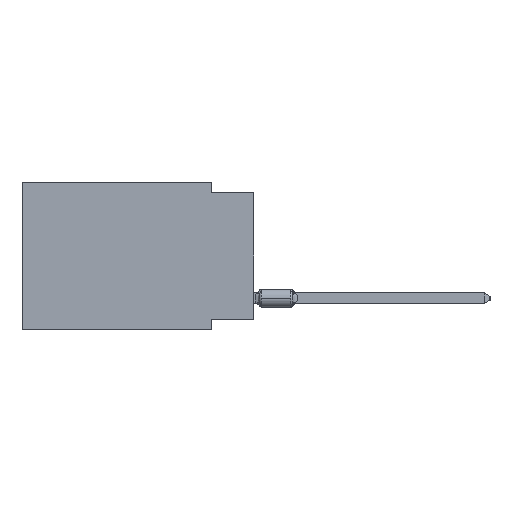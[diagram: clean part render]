
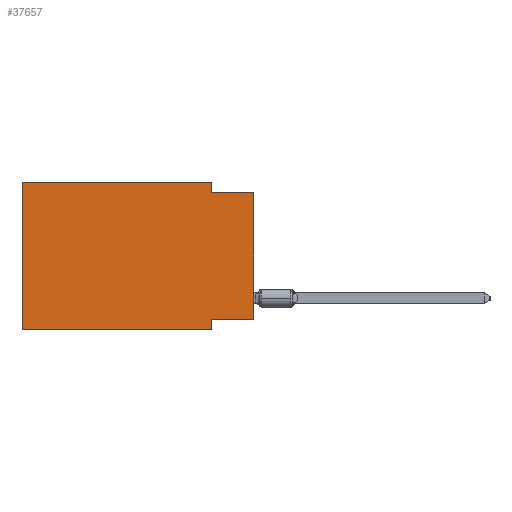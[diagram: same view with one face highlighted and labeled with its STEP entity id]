
A CAD part, left-side view. The second image highlights one B-rep face of the part: STEP entity #37657.
In plain terms, the highlighted planar face has unit normal (-1, 0, 0).
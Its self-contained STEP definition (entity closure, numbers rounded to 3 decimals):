
#458 = EDGE_CURVE ( 'NONE', #14854, #29812, #41753, .T. ) ;
#502 = ORIENTED_EDGE ( 'NONE', *, *, #43534, .T. ) ;
#1243 = CARTESIAN_POINT ( 'NONE',  ( 0., 2.54, -8.255 ) ) ;
#1617 = LINE ( 'NONE', #15520, #10280 ) ;
#2071 = VECTOR ( 'NONE', #35717, 1000. ) ;
#2392 = VERTEX_POINT ( 'NONE', #25426 ) ;
#7444 = VECTOR ( 'NONE', #23663, 1000. ) ;
#8389 = EDGE_CURVE ( 'NONE', #2392, #30727, #14207, .T. ) ;
#8880 = ORIENTED_EDGE ( 'NONE', *, *, #15803, .T. ) ;
#9015 = VECTOR ( 'NONE', #29003, 1000. ) ;
#9169 = VERTEX_POINT ( 'NONE', #44141 ) ;
#9697 = VERTEX_POINT ( 'NONE', #14405 ) ;
#10077 = CARTESIAN_POINT ( 'NONE',  ( 0., 0., -0.635 ) ) ;
#10280 = VECTOR ( 'NONE', #29429, 1000. ) ;
#10517 = CARTESIAN_POINT ( 'NONE',  ( 0., 2.54, -8.89 ) ) ;
#11199 = ORIENTED_EDGE ( 'NONE', *, *, #38342, .F. ) ;
#11310 = DIRECTION ( 'NONE',  ( 1., 0., 0. ) ) ;
#11947 = VERTEX_POINT ( 'NONE', #10077 ) ;
#12140 = DIRECTION ( 'NONE',  ( 0., 0., -1. ) ) ;
#12827 = ORIENTED_EDGE ( 'NONE', *, *, #37064, .F. ) ;
#14122 = VERTEX_POINT ( 'NONE', #43372 ) ;
#14207 = LINE ( 'NONE', #21698, #28660 ) ;
#14405 = CARTESIAN_POINT ( 'NONE',  ( 0., 13.97, -8.89 ) ) ;
#14854 = VERTEX_POINT ( 'NONE', #1243 ) ;
#15520 = CARTESIAN_POINT ( 'NONE',  ( 0., 13.97, 0. ) ) ;
#15803 = EDGE_CURVE ( 'NONE', #9697, #29812, #36028, .T. ) ;
#16454 = LINE ( 'NONE', #16675, #33556 ) ;
#16675 = CARTESIAN_POINT ( 'NONE',  ( 0., 0., -8.255 ) ) ;
#17127 = DIRECTION ( 'NONE',  ( 0., 0., -1. ) ) ;
#18142 = LINE ( 'NONE', #42327, #2071 ) ;
#18324 = ORIENTED_EDGE ( 'NONE', *, *, #38640, .F. ) ;
#18485 = ORIENTED_EDGE ( 'NONE', *, *, #458, .F. ) ;
#18535 = LINE ( 'NONE', #32450, #9015 ) ;
#20861 = DIRECTION ( 'NONE',  ( 0., 0., -1. ) ) ;
#21121 = AXIS2_PLACEMENT_3D ( 'NONE', #28156, #11310, #20861 ) ;
#21698 = CARTESIAN_POINT ( 'NONE',  ( 0., 13.97, 0. ) ) ;
#22496 = VECTOR ( 'NONE', #17127, 1000. ) ;
#23663 = DIRECTION ( 'NONE',  ( 0., -1., 0. ) ) ;
#23718 = CARTESIAN_POINT ( 'NONE',  ( 0., 2.54, -8.89 ) ) ;
#23875 = CARTESIAN_POINT ( 'NONE',  ( 0., 13.97, -8.89 ) ) ;
#25283 = ORIENTED_EDGE ( 'NONE', *, *, #8389, .F. ) ;
#25426 = CARTESIAN_POINT ( 'NONE',  ( 0., 13.97, 0. ) ) ;
#25676 = EDGE_CURVE ( 'NONE', #14122, #11947, #18142, .T. ) ;
#28098 = DIRECTION ( 'NONE',  ( 0., -1., 0. ) ) ;
#28156 = CARTESIAN_POINT ( 'NONE',  ( 0., 13.97, 0. ) ) ;
#28660 = VECTOR ( 'NONE', #28098, 1000. ) ;
#29003 = DIRECTION ( 'NONE',  ( 0., 0., 1. ) ) ;
#29429 = DIRECTION ( 'NONE',  ( 0., 0., 1. ) ) ;
#29812 = VERTEX_POINT ( 'NONE', #23718 ) ;
#30239 = CARTESIAN_POINT ( 'NONE',  ( 0., 2.54, 0. ) ) ;
#30727 = VERTEX_POINT ( 'NONE', #30239 ) ;
#32450 = CARTESIAN_POINT ( 'NONE',  ( 0., 0., 0. ) ) ;
#32746 = VECTOR ( 'NONE', #12140, 1000. ) ;
#33556 = VECTOR ( 'NONE', #37219, 1000. ) ;
#35479 = PLANE ( 'NONE',  #21121 ) ;
#35717 = DIRECTION ( 'NONE',  ( 0., -1., 0. ) ) ;
#36028 = LINE ( 'NONE', #23875, #7444 ) ;
#37064 = EDGE_CURVE ( 'NONE', #30727, #14122, #42707, .T. ) ;
#37219 = DIRECTION ( 'NONE',  ( 0., 1., 0. ) ) ;
#37657 = ADVANCED_FACE ( 'NONE', ( #39128 ), #35479, .F. ) ;
#38342 = EDGE_CURVE ( 'NONE', #9169, #14854, #16454, .T. ) ;
#38640 = EDGE_CURVE ( 'NONE', #9697, #2392, #1617, .T. ) ;
#39128 = FACE_OUTER_BOUND ( 'NONE', #40402, .T. ) ;
#39741 = CARTESIAN_POINT ( 'NONE',  ( 0., 2.54, 0. ) ) ;
#40402 = EDGE_LOOP ( 'NONE', ( #502, #44742, #12827, #25283, #18324, #8880, #18485, #11199 ) ) ;
#41753 = LINE ( 'NONE', #10517, #22496 ) ;
#42327 = CARTESIAN_POINT ( 'NONE',  ( 0., 0., -0.635 ) ) ;
#42707 = LINE ( 'NONE', #39741, #32746 ) ;
#43372 = CARTESIAN_POINT ( 'NONE',  ( 0., 2.54, -0.635 ) ) ;
#43534 = EDGE_CURVE ( 'NONE', #9169, #11947, #18535, .T. ) ;
#44141 = CARTESIAN_POINT ( 'NONE',  ( 0., 0., -8.255 ) ) ;
#44742 = ORIENTED_EDGE ( 'NONE', *, *, #25676, .F. ) ;
